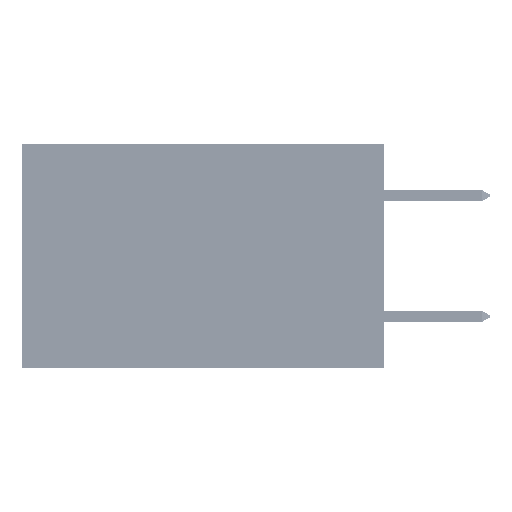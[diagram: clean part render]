
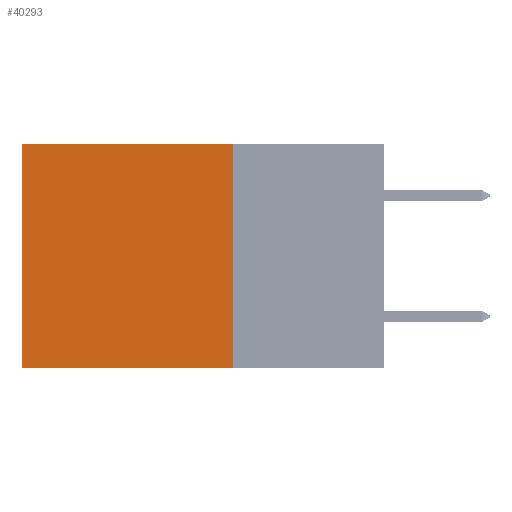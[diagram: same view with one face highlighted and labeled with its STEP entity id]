
A CAD part, left-side view. The second image highlights one B-rep face of the part: STEP entity #40293.
In plain terms, the highlighted planar face has unit normal (-1, 0, 0).
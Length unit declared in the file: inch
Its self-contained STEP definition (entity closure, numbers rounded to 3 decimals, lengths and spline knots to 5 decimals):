
#1358 = FACE_OUTER_BOUND ( 'NONE', #48508, .T. ) ;
#1575 = VECTOR ( 'NONE', #45932, 39.37008 ) ;
#9240 = DIRECTION ( 'NONE',  ( 0., 0., -1. ) ) ;
#9894 = ORIENTED_EDGE ( 'NONE', *, *, #37406, .T. ) ;
#11138 = CARTESIAN_POINT ( 'NONE',  ( 0.2875, 0.6, -0.37 ) ) ;
#12619 = CARTESIAN_POINT ( 'NONE',  ( 0.2875, 0.25, 0. ) ) ;
#13928 = AXIS2_PLACEMENT_3D ( 'NONE', #12619, #47358, #9240 ) ;
#14309 = ORIENTED_EDGE ( 'NONE', *, *, #33344, .T. ) ;
#14983 = CARTESIAN_POINT ( 'NONE',  ( 0.2875, 0.6, 0. ) ) ;
#16134 = DIRECTION ( 'NONE',  ( 0., 0., -1. ) ) ;
#16524 = CARTESIAN_POINT ( 'NONE',  ( 0.2875, 0.25, 0. ) ) ;
#18451 = VERTEX_POINT ( 'NONE', #26835 ) ;
#18604 = ORIENTED_EDGE ( 'NONE', *, *, #43831, .F. ) ;
#19219 = LINE ( 'NONE', #26925, #28308 ) ;
#20623 = VERTEX_POINT ( 'NONE', #14983 ) ;
#23085 = EDGE_CURVE ( 'NONE', #18451, #47135, #38990, .T. ) ;
#23685 = DIRECTION ( 'NONE',  ( 0., 0., -1. ) ) ;
#26835 = CARTESIAN_POINT ( 'NONE',  ( 0.2875, 0.25, -0.37 ) ) ;
#26925 = CARTESIAN_POINT ( 'NONE',  ( 0.2875, 0.6, 0. ) ) ;
#28308 = VECTOR ( 'NONE', #23685, 39.37008 ) ;
#30423 = DIRECTION ( 'NONE',  ( 0., 1., 0. ) ) ;
#31795 = LINE ( 'NONE', #42019, #46246 ) ;
#33344 = EDGE_CURVE ( 'NONE', #37674, #20623, #31795, .T. ) ;
#34003 = ORIENTED_EDGE ( 'NONE', *, *, #23085, .F. ) ;
#35374 = CARTESIAN_POINT ( 'NONE',  ( 0.2875, 0.25, 0. ) ) ;
#37406 = EDGE_CURVE ( 'NONE', #20623, #47135, #19219, .T. ) ;
#37674 = VERTEX_POINT ( 'NONE', #16524 ) ;
#38990 = LINE ( 'NONE', #45614, #1575 ) ;
#39621 = LINE ( 'NONE', #35374, #43221 ) ;
#40293 = ADVANCED_FACE ( 'NONE', ( #1358 ), #47864, .F. ) ;
#42019 = CARTESIAN_POINT ( 'NONE',  ( 0.2875, 0.25, 0. ) ) ;
#43221 = VECTOR ( 'NONE', #16134, 39.37008 ) ;
#43831 = EDGE_CURVE ( 'NONE', #37674, #18451, #39621, .T. ) ;
#45614 = CARTESIAN_POINT ( 'NONE',  ( 0.2875, 0.25, -0.37 ) ) ;
#45932 = DIRECTION ( 'NONE',  ( 0., 1., 0. ) ) ;
#46246 = VECTOR ( 'NONE', #30423, 39.37008 ) ;
#47135 = VERTEX_POINT ( 'NONE', #11138 ) ;
#47358 = DIRECTION ( 'NONE',  ( 1., 0., 0. ) ) ;
#47864 = PLANE ( 'NONE',  #13928 ) ;
#48508 = EDGE_LOOP ( 'NONE', ( #9894, #34003, #18604, #14309 ) ) ;
